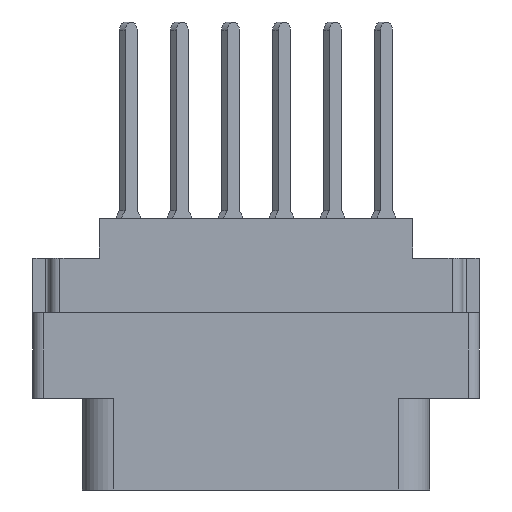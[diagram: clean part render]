
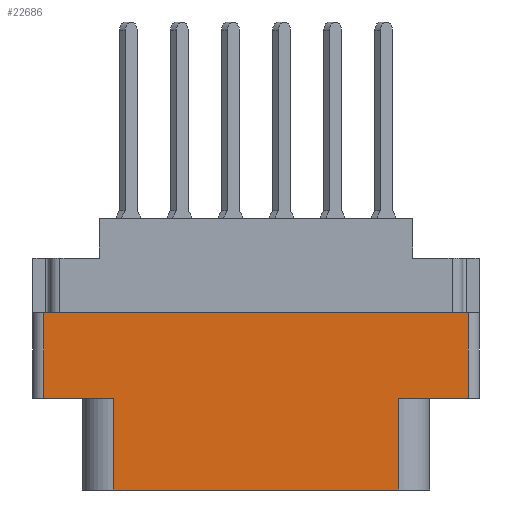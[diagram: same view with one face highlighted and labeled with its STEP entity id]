
A CAD part, front view. The second image highlights one B-rep face of the part: STEP entity #22686.
In plain terms, the highlighted planar face has unit normal (0, -1, 0).
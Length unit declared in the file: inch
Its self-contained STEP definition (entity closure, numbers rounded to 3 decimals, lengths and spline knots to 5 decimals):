
#341 = ORIENTED_EDGE ( 'NONE', *, *, #7363, .F. ) ;
#854 = VECTOR ( 'NONE', #24203, 39.37008 ) ;
#908 = EDGE_CURVE ( 'NONE', #8511, #21515, #18155, .T. ) ;
#1043 = ORIENTED_EDGE ( 'NONE', *, *, #17156, .F. ) ;
#2064 = DIRECTION ( 'NONE',  ( 0., 0., 1. ) ) ;
#2358 = LINE ( 'NONE', #20223, #19049 ) ;
#2639 = ORIENTED_EDGE ( 'NONE', *, *, #22405, .T. ) ;
#2773 = VERTEX_POINT ( 'NONE', #2809 ) ;
#2809 = CARTESIAN_POINT ( 'NONE',  ( -0.42, -0.343, -0.798 ) ) ;
#3116 = EDGE_CURVE ( 'NONE', #15556, #17441, #4588, .T. ) ;
#3117 = LINE ( 'NONE', #23247, #18926 ) ;
#4040 = EDGE_CURVE ( 'NONE', #15556, #21019, #3117, .T. ) ;
#4084 = CARTESIAN_POINT ( 'NONE',  ( 0.42, -0.343, -0.798 ) ) ;
#4378 = EDGE_LOOP ( 'NONE', ( #2639, #15872, #1043, #20717, #19150, #7746, #341, #22646 ) ) ;
#4567 = VECTOR ( 'NONE', #2064, 39.37008 ) ;
#4588 = LINE ( 'NONE', #14980, #4567 ) ;
#5047 = VECTOR ( 'NONE', #8651, 39.37008 ) ;
#5108 = DIRECTION ( 'NONE',  ( -1., 0., 0. ) ) ;
#5344 = CARTESIAN_POINT ( 'NONE',  ( -0.42, -0.343, -0.529 ) ) ;
#6487 = LINE ( 'NONE', #8488, #5047 ) ;
#6527 = CARTESIAN_POINT ( 'NONE',  ( -0.624, -0.343, -0.798 ) ) ;
#7239 = EDGE_CURVE ( 'NONE', #2773, #14514, #8252, .T. ) ;
#7337 = EDGE_CURVE ( 'NONE', #10609, #17441, #6487, .T. ) ;
#7363 = EDGE_CURVE ( 'NONE', #8511, #10609, #8844, .T. ) ;
#7746 = ORIENTED_EDGE ( 'NONE', *, *, #7337, .F. ) ;
#8020 = DIRECTION ( 'NONE',  ( 0., -1., 0. ) ) ;
#8252 = LINE ( 'NONE', #9913, #24027 ) ;
#8263 = PLANE ( 'NONE',  #12236 ) ;
#8488 = CARTESIAN_POINT ( 'NONE',  ( -0.656, -0.343, -0.277 ) ) ;
#8511 = VERTEX_POINT ( 'NONE', #20618 ) ;
#8651 = DIRECTION ( 'NONE',  ( 1., 0., 0. ) ) ;
#8844 = LINE ( 'NONE', #6527, #21435 ) ;
#9004 = DIRECTION ( 'NONE',  ( 0., 0., -1. ) ) ;
#9913 = CARTESIAN_POINT ( 'NONE',  ( -0.624, -0.343, -0.798 ) ) ;
#10609 = VERTEX_POINT ( 'NONE', #19516 ) ;
#11800 = DIRECTION ( 'NONE',  ( 0., 0., -1. ) ) ;
#12236 = AXIS2_PLACEMENT_3D ( 'NONE', #21365, #8020, #11800 ) ;
#12528 = LINE ( 'NONE', #5344, #854 ) ;
#12551 = CARTESIAN_POINT ( 'NONE',  ( 0.624, -0.343, -0.529 ) ) ;
#14221 = CARTESIAN_POINT ( 'NONE',  ( 0.624, -0.343, -0.277 ) ) ;
#14349 = CARTESIAN_POINT ( 'NONE',  ( 0., -0.343, -0.529 ) ) ;
#14514 = VERTEX_POINT ( 'NONE', #4084 ) ;
#14980 = CARTESIAN_POINT ( 'NONE',  ( 0.624, -0.343, -0.798 ) ) ;
#15556 = VERTEX_POINT ( 'NONE', #12551 ) ;
#15603 = CARTESIAN_POINT ( 'NONE',  ( -0.42, -0.343, -0.529 ) ) ;
#15872 = ORIENTED_EDGE ( 'NONE', *, *, #7239, .T. ) ;
#17156 = EDGE_CURVE ( 'NONE', #21019, #14514, #2358, .T. ) ;
#17441 = VERTEX_POINT ( 'NONE', #14221 ) ;
#18000 = DIRECTION ( 'NONE',  ( 0., 0., 1. ) ) ;
#18056 = DIRECTION ( 'NONE',  ( 1., 0., 0. ) ) ;
#18155 = LINE ( 'NONE', #14349, #21646 ) ;
#18926 = VECTOR ( 'NONE', #5108, 39.37008 ) ;
#19049 = VECTOR ( 'NONE', #9004, 39.37008 ) ;
#19150 = ORIENTED_EDGE ( 'NONE', *, *, #3116, .T. ) ;
#19516 = CARTESIAN_POINT ( 'NONE',  ( -0.624, -0.343, -0.277 ) ) ;
#19561 = FACE_OUTER_BOUND ( 'NONE', #4378, .T. ) ;
#20223 = CARTESIAN_POINT ( 'NONE',  ( 0.42, -0.343, -0.529 ) ) ;
#20618 = CARTESIAN_POINT ( 'NONE',  ( -0.624, -0.343, -0.529 ) ) ;
#20717 = ORIENTED_EDGE ( 'NONE', *, *, #4040, .F. ) ;
#21019 = VERTEX_POINT ( 'NONE', #21202 ) ;
#21202 = CARTESIAN_POINT ( 'NONE',  ( 0.42, -0.343, -0.529 ) ) ;
#21365 = CARTESIAN_POINT ( 'NONE',  ( -0.624, -0.343, -0.798 ) ) ;
#21435 = VECTOR ( 'NONE', #18000, 39.37008 ) ;
#21515 = VERTEX_POINT ( 'NONE', #15603 ) ;
#21646 = VECTOR ( 'NONE', #18056, 39.37008 ) ;
#22405 = EDGE_CURVE ( 'NONE', #21515, #2773, #12528, .T. ) ;
#22646 = ORIENTED_EDGE ( 'NONE', *, *, #908, .T. ) ;
#22686 = ADVANCED_FACE ( 'NONE', ( #19561 ), #8263, .T. ) ;
#22972 = DIRECTION ( 'NONE',  ( 1., 0., 0. ) ) ;
#23247 = CARTESIAN_POINT ( 'NONE',  ( 0., -0.343, -0.529 ) ) ;
#24027 = VECTOR ( 'NONE', #22972, 39.37008 ) ;
#24203 = DIRECTION ( 'NONE',  ( 0., 0., -1. ) ) ;
